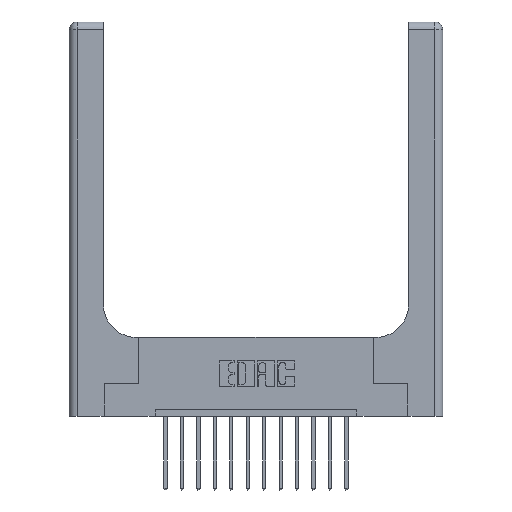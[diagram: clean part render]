
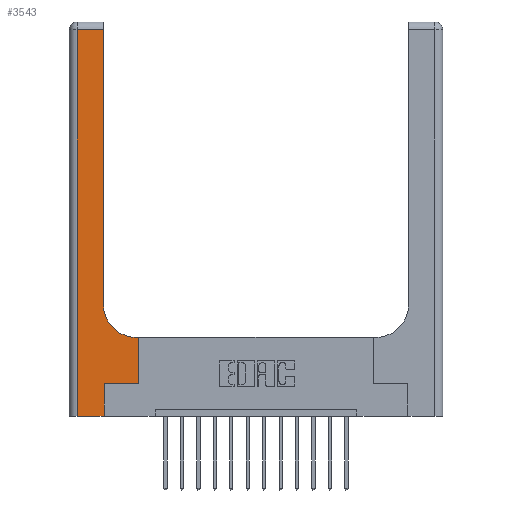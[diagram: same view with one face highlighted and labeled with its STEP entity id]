
A CAD part, top view. The second image highlights one B-rep face of the part: STEP entity #3543.
In plain terms, the highlighted planar face has unit normal (0, 0, 1).
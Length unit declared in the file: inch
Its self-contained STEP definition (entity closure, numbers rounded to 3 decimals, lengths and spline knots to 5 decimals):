
#216 = CARTESIAN_POINT ( 'NONE',  ( 0.528, 0.25, 0.37 ) ) ;
#288 = CARTESIAN_POINT ( 'NONE',  ( 0.26, 0.6, 0.37 ) ) ;
#463 = LINE ( 'NONE', #10925, #9962 ) ;
#1083 = CARTESIAN_POINT ( 'NONE',  ( 0.26, 0.85, 0.37 ) ) ;
#1122 = ORIENTED_EDGE ( 'NONE', *, *, #3764, .T. ) ;
#1376 = EDGE_CURVE ( 'NONE', #4920, #8968, #15881, .T. ) ;
#1656 = EDGE_CURVE ( 'NONE', #4719, #7282, #3499, .T. ) ;
#1770 = LINE ( 'NONE', #13706, #10722 ) ;
#2112 = AXIS2_PLACEMENT_3D ( 'NONE', #15724, #9051, #3862 ) ;
#2711 = CARTESIAN_POINT ( 'NONE',  ( 0.06, 2.94, 0.37 ) ) ;
#2802 = CARTESIAN_POINT ( 'NONE',  ( 0.26, 3., 0.37 ) ) ;
#2806 = VERTEX_POINT ( 'NONE', #1083 ) ;
#3068 = LINE ( 'NONE', #15009, #4517 ) ;
#3499 = LINE ( 'NONE', #6251, #11862 ) ;
#3543 = ADVANCED_FACE ( 'NONE', ( #10165 ), #15534, .F. ) ;
#3580 = VECTOR ( 'NONE', #13447, 39.37008 ) ;
#3764 = EDGE_CURVE ( 'NONE', #7498, #8309, #463, .T. ) ;
#3821 = ORIENTED_EDGE ( 'NONE', *, *, #15447, .T. ) ;
#3862 = DIRECTION ( 'NONE',  ( 1., 0., 0. ) ) ;
#4109 = DIRECTION ( 'NONE',  ( 0., 1., 0. ) ) ;
#4111 = LINE ( 'NONE', #4275, #3580 ) ;
#4275 = CARTESIAN_POINT ( 'NONE',  ( 0.06, 3., 0.37 ) ) ;
#4302 = CARTESIAN_POINT ( 'NONE',  ( 0.265, 0.25, 0.37 ) ) ;
#4343 = CARTESIAN_POINT ( 'NONE',  ( 0.265, 0., 0.37 ) ) ;
#4517 = VECTOR ( 'NONE', #16664, 39.37008 ) ;
#4719 = VERTEX_POINT ( 'NONE', #15785 ) ;
#4882 = CIRCLE ( 'NONE', #2112, 0.25 ) ;
#4920 = VERTEX_POINT ( 'NONE', #5757 ) ;
#5757 = CARTESIAN_POINT ( 'NONE',  ( 0.528, 0.25, 0.37 ) ) ;
#6012 = CARTESIAN_POINT ( 'NONE',  ( 0., 3., 0.37 ) ) ;
#6251 = CARTESIAN_POINT ( 'NONE',  ( 0., 0., 0.37 ) ) ;
#6378 = EDGE_CURVE ( 'NONE', #8309, #4719, #4111, .T. ) ;
#6392 = ORIENTED_EDGE ( 'NONE', *, *, #1656, .T. ) ;
#6589 = LINE ( 'NONE', #2802, #14645 ) ;
#6927 = DIRECTION ( 'NONE',  ( 0., 1., 0. ) ) ;
#6952 = ORIENTED_EDGE ( 'NONE', *, *, #11127, .T. ) ;
#7282 = VERTEX_POINT ( 'NONE', #4343 ) ;
#7484 = VERTEX_POINT ( 'NONE', #4302 ) ;
#7498 = VERTEX_POINT ( 'NONE', #12095 ) ;
#7654 = DIRECTION ( 'NONE',  ( -1., 0., 0. ) ) ;
#8076 = EDGE_CURVE ( 'NONE', #7282, #7484, #3068, .T. ) ;
#8309 = VERTEX_POINT ( 'NONE', #2711 ) ;
#8968 = VERTEX_POINT ( 'NONE', #15569 ) ;
#9051 = DIRECTION ( 'NONE',  ( 0., 0., -1. ) ) ;
#9400 = AXIS2_PLACEMENT_3D ( 'NONE', #6012, #16762, #7654 ) ;
#9475 = EDGE_CURVE ( 'NONE', #8968, #14340, #15955, .T. ) ;
#9962 = VECTOR ( 'NONE', #16214, 39.37008 ) ;
#10165 = FACE_OUTER_BOUND ( 'NONE', #12195, .T. ) ;
#10722 = VECTOR ( 'NONE', #15098, 39.37008 ) ;
#10925 = CARTESIAN_POINT ( 'NONE',  ( 0., 2.94, 0.37 ) ) ;
#10932 = ORIENTED_EDGE ( 'NONE', *, *, #16988, .T. ) ;
#11127 = EDGE_CURVE ( 'NONE', #14340, #2806, #4882, .T. ) ;
#11541 = DIRECTION ( 'NONE',  ( 1., 0., 0. ) ) ;
#11862 = VECTOR ( 'NONE', #11541, 39.37008 ) ;
#11972 = DIRECTION ( 'NONE',  ( -1., 0., 0. ) ) ;
#12095 = CARTESIAN_POINT ( 'NONE',  ( 0.26, 2.94, 0.37 ) ) ;
#12195 = EDGE_LOOP ( 'NONE', ( #10932, #1122, #14168, #6392, #12257, #3821, #13381, #14766, #6952 ) ) ;
#12257 = ORIENTED_EDGE ( 'NONE', *, *, #8076, .T. ) ;
#12404 = CARTESIAN_POINT ( 'NONE',  ( 0.51, 0.6, 0.37 ) ) ;
#13381 = ORIENTED_EDGE ( 'NONE', *, *, #1376, .T. ) ;
#13447 = DIRECTION ( 'NONE',  ( 0., -1., 0. ) ) ;
#13706 = CARTESIAN_POINT ( 'NONE',  ( 0.265, 0.25, 0.37 ) ) ;
#14168 = ORIENTED_EDGE ( 'NONE', *, *, #6378, .T. ) ;
#14340 = VERTEX_POINT ( 'NONE', #12404 ) ;
#14645 = VECTOR ( 'NONE', #6927, 39.37008 ) ;
#14766 = ORIENTED_EDGE ( 'NONE', *, *, #9475, .T. ) ;
#15009 = CARTESIAN_POINT ( 'NONE',  ( 0.265, 0., 0.37 ) ) ;
#15069 = VECTOR ( 'NONE', #4109, 39.37008 ) ;
#15098 = DIRECTION ( 'NONE',  ( 1., 0., 0. ) ) ;
#15447 = EDGE_CURVE ( 'NONE', #7484, #4920, #1770, .T. ) ;
#15534 = PLANE ( 'NONE',  #9400 ) ;
#15569 = CARTESIAN_POINT ( 'NONE',  ( 0.528, 0.6, 0.37 ) ) ;
#15724 = CARTESIAN_POINT ( 'NONE',  ( 0.51, 0.85, 0.37 ) ) ;
#15785 = CARTESIAN_POINT ( 'NONE',  ( 0.06, 0., 0.37 ) ) ;
#15881 = LINE ( 'NONE', #216, #15069 ) ;
#15955 = LINE ( 'NONE', #288, #16169 ) ;
#16169 = VECTOR ( 'NONE', #11972, 39.37008 ) ;
#16214 = DIRECTION ( 'NONE',  ( -1., 0., 0. ) ) ;
#16664 = DIRECTION ( 'NONE',  ( 0., 1., 0. ) ) ;
#16762 = DIRECTION ( 'NONE',  ( 0., 0., -1. ) ) ;
#16988 = EDGE_CURVE ( 'NONE', #2806, #7498, #6589, .T. ) ;
